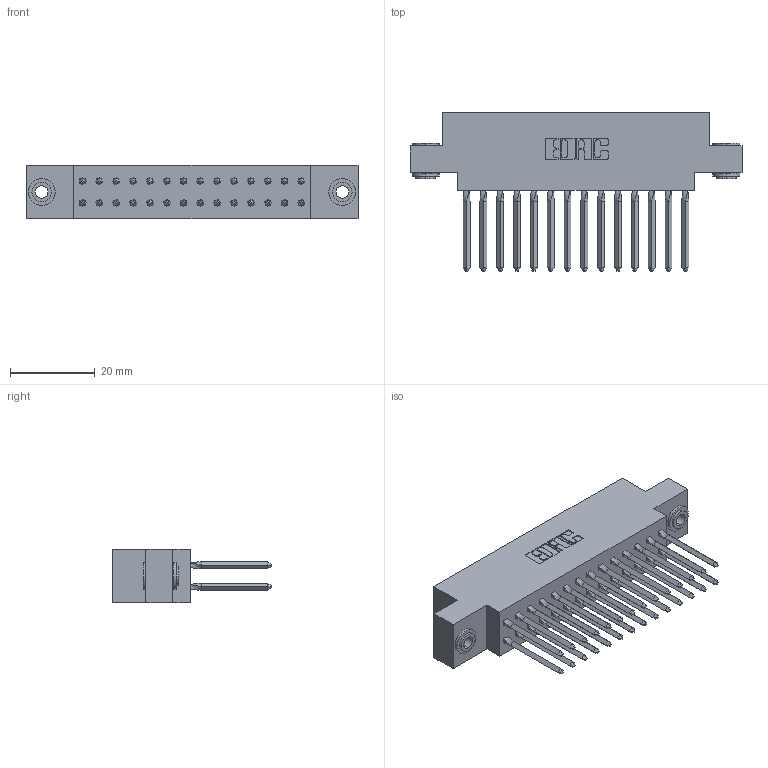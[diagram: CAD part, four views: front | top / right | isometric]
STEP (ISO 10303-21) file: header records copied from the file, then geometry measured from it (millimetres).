
FILE_DESCRIPTION (( 'STEP AP203' ), '1' );
FILE_NAME ('317-028-542-803.STEP', '2020-02-27T19:40:18', ( '' ), ( '' ), 'SwSTEP 2.0', 'SolidWorks 2016', '' );
FILE_SCHEMA (( 'CONFIG_CONTROL_DESIGN' ));
Length unit declared in the file: inch
Products named in the file (4): 345-250-002_345-250-002-102; 317-290-003_542; 317 Part_.156 Dia - TH; 317-028-542-803
Assembly tree (31 placements, depth 2):
  317-028-542-803
    317 Part_.156 Dia - TH
    317-290-003_542  x28
    345-250-002_345-250-002-102  x2
Bounding box: 78.18 x 37.34 x 12.7 mm (x, y, z)
Volume: 11936.4 mm3; surface area: 15916.5 mm2
Topology: 31 solids, 31 shells, 1736 faces, 4831 edges, 3086 vertices
Faces by surface type: plane 1356, cylinder 260, bspline 112, cone 8
Entity records: 23810 total; most frequent: CARTESIAN_POINT 4368, ORIENTED_EDGE 4024, DIRECTION 3474, EDGE_CURVE 2012, VECTOR 1818, LINE 1818, VERTEX_POINT 1334, AXIS2_PLACEMENT_3D 828
